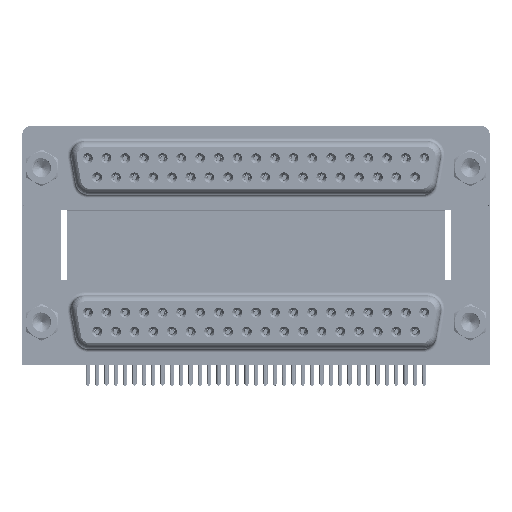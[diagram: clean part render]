
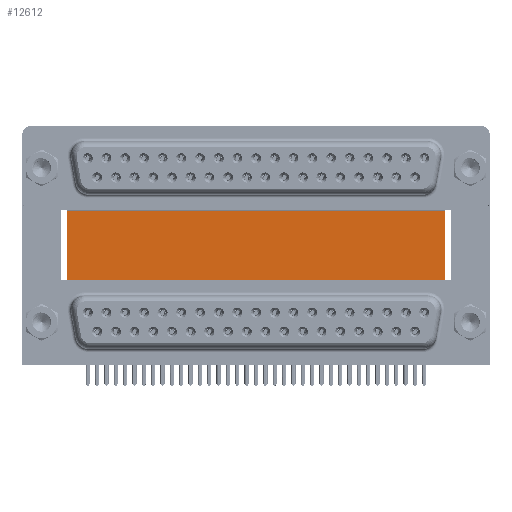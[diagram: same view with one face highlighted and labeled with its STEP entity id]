
A CAD part, top view. The second image highlights one B-rep face of the part: STEP entity #12612.
In plain terms, the highlighted planar face has unit normal (0, 0, 1).
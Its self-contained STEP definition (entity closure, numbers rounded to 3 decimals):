
#1134 = FACE_OUTER_BOUND ( 'NONE', #69615, .T. ) ;
#11236 = LINE ( 'NONE', #63319, #15167 ) ;
#12478 = CARTESIAN_POINT ( 'NONE',  ( 3.79, 16.585, -12. ) ) ;
#12612 = ADVANCED_FACE ( 'NONE', ( #1134 ), #44981, .F. ) ;
#12642 = CARTESIAN_POINT ( 'NONE',  ( 59.71, 16.585, -12. ) ) ;
#13158 = ORIENTED_EDGE ( 'NONE', *, *, #31587, .T. ) ;
#15167 = VECTOR ( 'NONE', #38102, 1000. ) ;
#15581 = AXIS2_PLACEMENT_3D ( 'NONE', #63183, #62777, #26373 ) ;
#26373 = DIRECTION ( 'NONE',  ( -1., 0., 0. ) ) ;
#30303 = EDGE_CURVE ( 'NONE', #53882, #55041, #32872, .T. ) ;
#30952 = CARTESIAN_POINT ( 'NONE',  ( 3.79, -3.735, -12. ) ) ;
#31587 = EDGE_CURVE ( 'NONE', #60080, #55933, #11236, .T. ) ;
#32213 = ORIENTED_EDGE ( 'NONE', *, *, #30303, .F. ) ;
#32872 = LINE ( 'NONE', #50262, #47923 ) ;
#38102 = DIRECTION ( 'NONE',  ( 1., 0., 0. ) ) ;
#40253 = EDGE_CURVE ( 'NONE', #53882, #60080, #64589, .T. ) ;
#44981 = PLANE ( 'NONE',  #15581 ) ;
#45825 = CARTESIAN_POINT ( 'NONE',  ( 3.79, 16.585, -12. ) ) ;
#47923 = VECTOR ( 'NONE', #57289, 1000. ) ;
#50262 = CARTESIAN_POINT ( 'NONE',  ( 3.79, 16.585, -12. ) ) ;
#52535 = ORIENTED_EDGE ( 'NONE', *, *, #71233, .F. ) ;
#53882 = VERTEX_POINT ( 'NONE', #45825 ) ;
#55041 = VERTEX_POINT ( 'NONE', #60972 ) ;
#55439 = ORIENTED_EDGE ( 'NONE', *, *, #40253, .T. ) ;
#55933 = VERTEX_POINT ( 'NONE', #75591 ) ;
#57289 = DIRECTION ( 'NONE',  ( 1., 0., 0. ) ) ;
#57867 = VECTOR ( 'NONE', #71678, 1000. ) ;
#58871 = LINE ( 'NONE', #12642, #57867 ) ;
#60080 = VERTEX_POINT ( 'NONE', #30952 ) ;
#60972 = CARTESIAN_POINT ( 'NONE',  ( 59.71, 16.585, -12. ) ) ;
#62777 = DIRECTION ( 'NONE',  ( 0., 0., -1. ) ) ;
#63183 = CARTESIAN_POINT ( 'NONE',  ( 3.79, 16.585, -12. ) ) ;
#63319 = CARTESIAN_POINT ( 'NONE',  ( 3.79, -3.735, -12. ) ) ;
#63761 = DIRECTION ( 'NONE',  ( 0., -1., 0. ) ) ;
#64589 = LINE ( 'NONE', #12478, #65527 ) ;
#65527 = VECTOR ( 'NONE', #63761, 1000. ) ;
#69615 = EDGE_LOOP ( 'NONE', ( #13158, #52535, #32213, #55439 ) ) ;
#71233 = EDGE_CURVE ( 'NONE', #55041, #55933, #58871, .T. ) ;
#71678 = DIRECTION ( 'NONE',  ( 0., -1., 0. ) ) ;
#75591 = CARTESIAN_POINT ( 'NONE',  ( 59.71, -3.735, -12. ) ) ;
